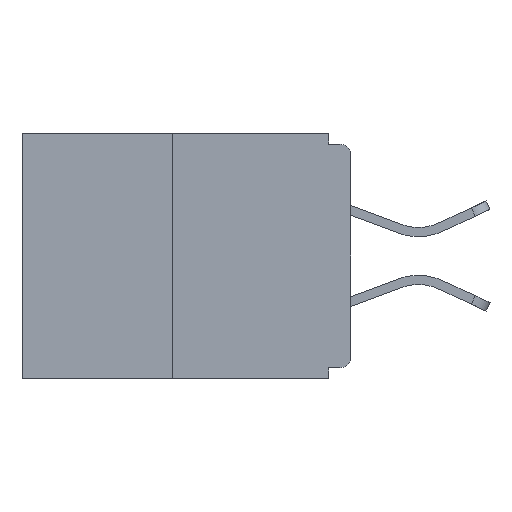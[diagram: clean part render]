
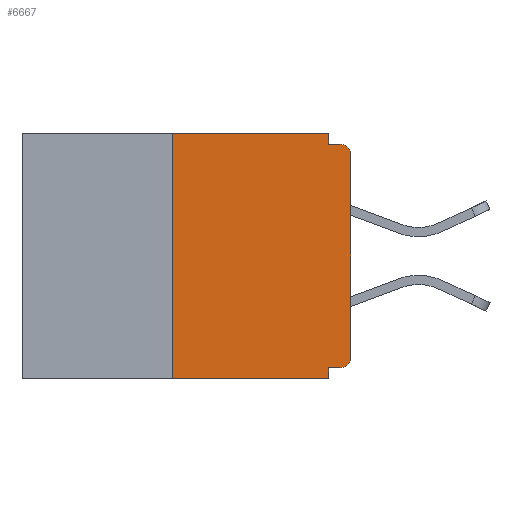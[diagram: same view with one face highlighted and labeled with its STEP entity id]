
A CAD part, left-side view. The second image highlights one B-rep face of the part: STEP entity #6667.
In plain terms, the highlighted planar face has unit normal (-1, 0, 0).
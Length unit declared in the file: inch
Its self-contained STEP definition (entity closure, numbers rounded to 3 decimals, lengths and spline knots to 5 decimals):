
#102 = CARTESIAN_POINT ( 'NONE',  ( 0., 0.015, -0.03 ) ) ;
#212 = EDGE_CURVE ( 'NONE', #17165, #15876, #7679, .T. ) ;
#242 = ORIENTED_EDGE ( 'NONE', *, *, #8488, .T. ) ;
#313 = EDGE_CURVE ( 'NONE', #4986, #2309, #9324, .T. ) ;
#907 = DIRECTION ( 'NONE',  ( -1., 0., 0. ) ) ;
#1540 = CARTESIAN_POINT ( 'NONE',  ( 0., 0.25, 0. ) ) ;
#1581 = LINE ( 'NONE', #14746, #8855 ) ;
#1712 = DIRECTION ( 'NONE',  ( 0., 0., -1. ) ) ;
#1761 = EDGE_CURVE ( 'NONE', #2309, #14514, #1581, .T. ) ;
#2309 = VERTEX_POINT ( 'NONE', #5828 ) ;
#2546 = ORIENTED_EDGE ( 'NONE', *, *, #11820, .F. ) ;
#2636 = VECTOR ( 'NONE', #5443, 39.37008 ) ;
#2884 = DIRECTION ( 'NONE',  ( 0., -1., 0. ) ) ;
#3063 = LINE ( 'NONE', #1540, #2636 ) ;
#3166 = EDGE_CURVE ( 'NONE', #15876, #16368, #15129, .T. ) ;
#3534 = DIRECTION ( 'NONE',  ( 0., -1., 0. ) ) ;
#3809 = CARTESIAN_POINT ( 'NONE',  ( 0., 0.46, 0. ) ) ;
#3853 = AXIS2_PLACEMENT_3D ( 'NONE', #8861, #907, #6273 ) ;
#3930 = EDGE_LOOP ( 'NONE', ( #16398, #8427, #6250, #2546, #4336, #242, #8536, #13726, #9363, #16507 ) ) ;
#4087 = FACE_OUTER_BOUND ( 'NONE', #3930, .T. ) ;
#4110 = VECTOR ( 'NONE', #13510, 39.37008 ) ;
#4112 = VERTEX_POINT ( 'NONE', #6990 ) ;
#4336 = ORIENTED_EDGE ( 'NONE', *, *, #14968, .F. ) ;
#4717 = EDGE_CURVE ( 'NONE', #14514, #16368, #12116, .T. ) ;
#4966 = AXIS2_PLACEMENT_3D ( 'NONE', #3809, #13198, #7979 ) ;
#4986 = VERTEX_POINT ( 'NONE', #13331 ) ;
#5029 = CIRCLE ( 'NONE', #3853, 0.015 ) ;
#5258 = DIRECTION ( 'NONE',  ( 0., 0., -1. ) ) ;
#5443 = DIRECTION ( 'NONE',  ( 0., 0., 1. ) ) ;
#5783 = LINE ( 'NONE', #14052, #10587 ) ;
#5801 = CARTESIAN_POINT ( 'NONE',  ( 0., 0., -0.03 ) ) ;
#5828 = CARTESIAN_POINT ( 'NONE',  ( 0., 0.031, 0. ) ) ;
#5838 = VECTOR ( 'NONE', #2884, 39.37008 ) ;
#5901 = VECTOR ( 'NONE', #14242, 39.37008 ) ;
#6097 = EDGE_CURVE ( 'NONE', #13516, #4986, #3063, .T. ) ;
#6250 = ORIENTED_EDGE ( 'NONE', *, *, #11698, .T. ) ;
#6273 = DIRECTION ( 'NONE',  ( 0., 0., -1. ) ) ;
#6523 = CARTESIAN_POINT ( 'NONE',  ( 0., 0.015, -0.015 ) ) ;
#6617 = VECTOR ( 'NONE', #6862, 39.37008 ) ;
#6667 = ADVANCED_FACE ( 'NONE', ( #4087 ), #16133, .F. ) ;
#6862 = DIRECTION ( 'NONE',  ( 0., -1., 0. ) ) ;
#6907 = CARTESIAN_POINT ( 'NONE',  ( 0., 0., 0. ) ) ;
#6990 = CARTESIAN_POINT ( 'NONE',  ( 0., 0.031, -0.343 ) ) ;
#7330 = DIRECTION ( 'NONE',  ( 0., 0., -1. ) ) ;
#7631 = CARTESIAN_POINT ( 'NONE',  ( 0., 0., -0.313 ) ) ;
#7679 = LINE ( 'NONE', #6907, #4110 ) ;
#7979 = DIRECTION ( 'NONE',  ( 0., 0., -1. ) ) ;
#8318 = VERTEX_POINT ( 'NONE', #15279 ) ;
#8427 = ORIENTED_EDGE ( 'NONE', *, *, #6097, .F. ) ;
#8488 = EDGE_CURVE ( 'NONE', #8318, #17165, #5029, .T. ) ;
#8536 = ORIENTED_EDGE ( 'NONE', *, *, #212, .T. ) ;
#8855 = VECTOR ( 'NONE', #5258, 39.37008 ) ;
#8861 = CARTESIAN_POINT ( 'NONE',  ( 0., 0.015, -0.313 ) ) ;
#9324 = LINE ( 'NONE', #10098, #12290 ) ;
#9363 = ORIENTED_EDGE ( 'NONE', *, *, #4717, .F. ) ;
#9907 = CARTESIAN_POINT ( 'NONE',  ( 0., 0.25, -0.343 ) ) ;
#10098 = CARTESIAN_POINT ( 'NONE',  ( 0., 0.46, 0. ) ) ;
#10276 = CARTESIAN_POINT ( 'NONE',  ( 0., 0.031, -0.015 ) ) ;
#10504 = LINE ( 'NONE', #13000, #5901 ) ;
#10520 = DIRECTION ( 'NONE',  ( -1., 0., 0. ) ) ;
#10587 = VECTOR ( 'NONE', #7330, 39.37008 ) ;
#10897 = CARTESIAN_POINT ( 'NONE',  ( 0., 0.46, -0.343 ) ) ;
#11698 = EDGE_CURVE ( 'NONE', #13516, #4112, #15025, .T. ) ;
#11820 = EDGE_CURVE ( 'NONE', #16080, #4112, #5783, .T. ) ;
#12116 = LINE ( 'NONE', #13588, #5838 ) ;
#12290 = VECTOR ( 'NONE', #3534, 39.37008 ) ;
#13000 = CARTESIAN_POINT ( 'NONE',  ( 0., 0., -0.328 ) ) ;
#13198 = DIRECTION ( 'NONE',  ( 1., 0., 0. ) ) ;
#13331 = CARTESIAN_POINT ( 'NONE',  ( 0., 0.25, 0. ) ) ;
#13510 = DIRECTION ( 'NONE',  ( 0., 0., 1. ) ) ;
#13516 = VERTEX_POINT ( 'NONE', #9907 ) ;
#13588 = CARTESIAN_POINT ( 'NONE',  ( 0., 0., -0.015 ) ) ;
#13726 = ORIENTED_EDGE ( 'NONE', *, *, #3166, .T. ) ;
#14052 = CARTESIAN_POINT ( 'NONE',  ( 0., 0.031, -0.343 ) ) ;
#14242 = DIRECTION ( 'NONE',  ( 0., 1., 0. ) ) ;
#14514 = VERTEX_POINT ( 'NONE', #10276 ) ;
#14746 = CARTESIAN_POINT ( 'NONE',  ( 0., 0.031, 0. ) ) ;
#14968 = EDGE_CURVE ( 'NONE', #8318, #16080, #10504, .T. ) ;
#15025 = LINE ( 'NONE', #10897, #6617 ) ;
#15129 = CIRCLE ( 'NONE', #16503, 0.015 ) ;
#15279 = CARTESIAN_POINT ( 'NONE',  ( 0., 0.015, -0.328 ) ) ;
#15876 = VERTEX_POINT ( 'NONE', #5801 ) ;
#16080 = VERTEX_POINT ( 'NONE', #16621 ) ;
#16133 = PLANE ( 'NONE',  #4966 ) ;
#16368 = VERTEX_POINT ( 'NONE', #6523 ) ;
#16398 = ORIENTED_EDGE ( 'NONE', *, *, #313, .F. ) ;
#16503 = AXIS2_PLACEMENT_3D ( 'NONE', #102, #10520, #1712 ) ;
#16507 = ORIENTED_EDGE ( 'NONE', *, *, #1761, .F. ) ;
#16621 = CARTESIAN_POINT ( 'NONE',  ( 0., 0.031, -0.328 ) ) ;
#17165 = VERTEX_POINT ( 'NONE', #7631 ) ;
